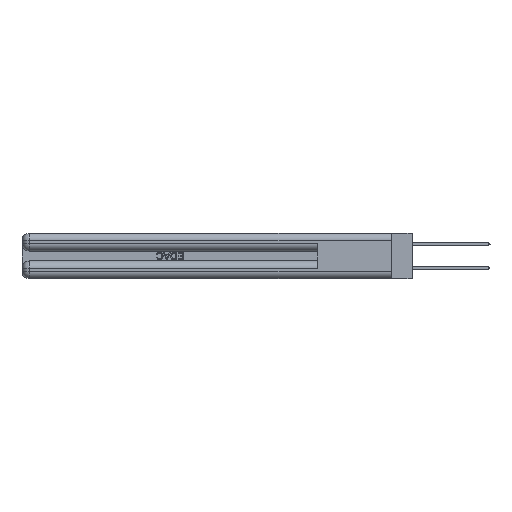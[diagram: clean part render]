
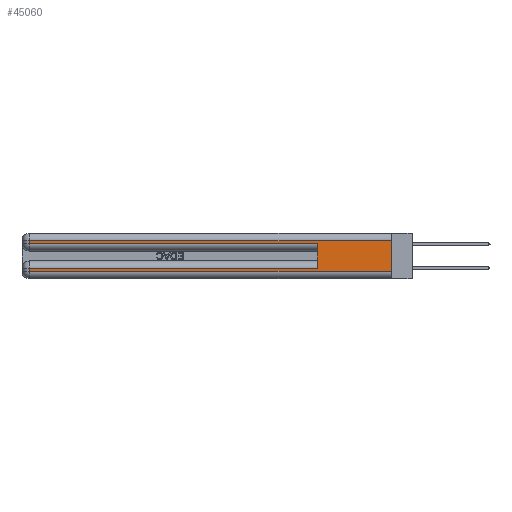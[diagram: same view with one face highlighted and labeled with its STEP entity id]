
A CAD part, left-side view. The second image highlights one B-rep face of the part: STEP entity #45060.
In plain terms, the highlighted planar face has unit normal (-1, 0, 0).
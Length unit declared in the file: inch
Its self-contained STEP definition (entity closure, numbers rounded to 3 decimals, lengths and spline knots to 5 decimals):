
#1297 = LINE ( 'NONE', #15234, #21087 ) ;
#2195 = VERTEX_POINT ( 'NONE', #7404 ) ;
#3610 = CARTESIAN_POINT ( 'NONE',  ( 0., 0., 0.31 ) ) ;
#3685 = EDGE_CURVE ( 'NONE', #15058, #2195, #1297, .T. ) ;
#4569 = LINE ( 'NONE', #3610, #13306 ) ;
#4965 = ORIENTED_EDGE ( 'NONE', *, *, #29256, .T. ) ;
#5189 = VERTEX_POINT ( 'NONE', #43498 ) ;
#5859 = VERTEX_POINT ( 'NONE', #35968 ) ;
#6629 = LINE ( 'NONE', #44246, #15354 ) ;
#7306 = ORIENTED_EDGE ( 'NONE', *, *, #3685, .F. ) ;
#7404 = CARTESIAN_POINT ( 'NONE',  ( 0., 0.6, 0.285 ) ) ;
#8023 = EDGE_CURVE ( 'NONE', #35350, #5189, #36690, .T. ) ;
#8454 = ORIENTED_EDGE ( 'NONE', *, *, #24571, .T. ) ;
#9888 = DIRECTION ( 'NONE',  ( 1., 0., 0. ) ) ;
#10642 = DIRECTION ( 'NONE',  ( 0., 0., -1. ) ) ;
#11550 = CARTESIAN_POINT ( 'NONE',  ( 0., 0., 0.06 ) ) ;
#11720 = CARTESIAN_POINT ( 'NONE',  ( 0., 0., 0.085 ) ) ;
#13306 = VECTOR ( 'NONE', #22152, 39.37008 ) ;
#13467 = PLANE ( 'NONE',  #46789 ) ;
#14995 = VECTOR ( 'NONE', #42090, 39.37008 ) ;
#15058 = VERTEX_POINT ( 'NONE', #22222 ) ;
#15234 = CARTESIAN_POINT ( 'NONE',  ( 0., 0.6, 0.145 ) ) ;
#15354 = VECTOR ( 'NONE', #22027, 39.37008 ) ;
#16590 = ORIENTED_EDGE ( 'NONE', *, *, #42011, .F. ) ;
#16963 = VECTOR ( 'NONE', #26542, 39.37008 ) ;
#17625 = VECTOR ( 'NONE', #39724, 39.37008 ) ;
#18796 = LINE ( 'NONE', #36002, #17625 ) ;
#20851 = EDGE_CURVE ( 'NONE', #5859, #41480, #27207, .T. ) ;
#21087 = VECTOR ( 'NONE', #41172, 39.37008 ) ;
#21487 = EDGE_LOOP ( 'NONE', ( #16590, #29950, #33404, #4965, #7306, #27086, #8454, #30541 ) ) ;
#22027 = DIRECTION ( 'NONE',  ( 0., 0., -1. ) ) ;
#22152 = DIRECTION ( 'NONE',  ( 0., 1., 0. ) ) ;
#22222 = CARTESIAN_POINT ( 'NONE',  ( 0., 0.6, 0.085 ) ) ;
#24571 = EDGE_CURVE ( 'NONE', #33602, #35350, #38439, .T. ) ;
#26542 = DIRECTION ( 'NONE',  ( 0., -1., 0. ) ) ;
#27086 = ORIENTED_EDGE ( 'NONE', *, *, #34459, .T. ) ;
#27207 = LINE ( 'NONE', #31060, #14995 ) ;
#28054 = LINE ( 'NONE', #11720, #40191 ) ;
#28500 = VERTEX_POINT ( 'NONE', #30170 ) ;
#29175 = CARTESIAN_POINT ( 'NONE',  ( 0., 2.94, 0.37 ) ) ;
#29256 = EDGE_CURVE ( 'NONE', #41480, #2195, #18796, .T. ) ;
#29950 = ORIENTED_EDGE ( 'NONE', *, *, #36385, .T. ) ;
#30170 = CARTESIAN_POINT ( 'NONE',  ( 0., 0., 0.31 ) ) ;
#30541 = ORIENTED_EDGE ( 'NONE', *, *, #8023, .T. ) ;
#31060 = CARTESIAN_POINT ( 'NONE',  ( 0., 2.94, 0.37 ) ) ;
#32104 = CARTESIAN_POINT ( 'NONE',  ( 0., 0., 0.37 ) ) ;
#33404 = ORIENTED_EDGE ( 'NONE', *, *, #20851, .T. ) ;
#33602 = VERTEX_POINT ( 'NONE', #47500 ) ;
#33932 = DIRECTION ( 'NONE',  ( 0., 1., 0. ) ) ;
#34459 = EDGE_CURVE ( 'NONE', #15058, #33602, #28054, .T. ) ;
#35350 = VERTEX_POINT ( 'NONE', #42184 ) ;
#35836 = DIRECTION ( 'NONE',  ( 0., 0., -1. ) ) ;
#35968 = CARTESIAN_POINT ( 'NONE',  ( 0., 2.94, 0.31 ) ) ;
#36002 = CARTESIAN_POINT ( 'NONE',  ( 0., 0., 0.285 ) ) ;
#36385 = EDGE_CURVE ( 'NONE', #28500, #5859, #4569, .T. ) ;
#36690 = LINE ( 'NONE', #11550, #16963 ) ;
#37277 = VECTOR ( 'NONE', #10642, 39.37008 ) ;
#38439 = LINE ( 'NONE', #29175, #37277 ) ;
#38899 = FACE_OUTER_BOUND ( 'NONE', #21487, .T. ) ;
#39724 = DIRECTION ( 'NONE',  ( 0., -1., 0. ) ) ;
#40191 = VECTOR ( 'NONE', #33932, 39.37008 ) ;
#41172 = DIRECTION ( 'NONE',  ( 0., 0., 1. ) ) ;
#41480 = VERTEX_POINT ( 'NONE', #45076 ) ;
#42011 = EDGE_CURVE ( 'NONE', #28500, #5189, #6629, .T. ) ;
#42090 = DIRECTION ( 'NONE',  ( 0., 0., -1. ) ) ;
#42184 = CARTESIAN_POINT ( 'NONE',  ( 0., 2.94, 0.06 ) ) ;
#43498 = CARTESIAN_POINT ( 'NONE',  ( 0., 0., 0.06 ) ) ;
#44246 = CARTESIAN_POINT ( 'NONE',  ( 0., 0., 0.37 ) ) ;
#45060 = ADVANCED_FACE ( 'NONE', ( #38899 ), #13467, .F. ) ;
#45076 = CARTESIAN_POINT ( 'NONE',  ( 0., 2.94, 0.285 ) ) ;
#46789 = AXIS2_PLACEMENT_3D ( 'NONE', #32104, #9888, #35836 ) ;
#47500 = CARTESIAN_POINT ( 'NONE',  ( 0., 2.94, 0.085 ) ) ;
